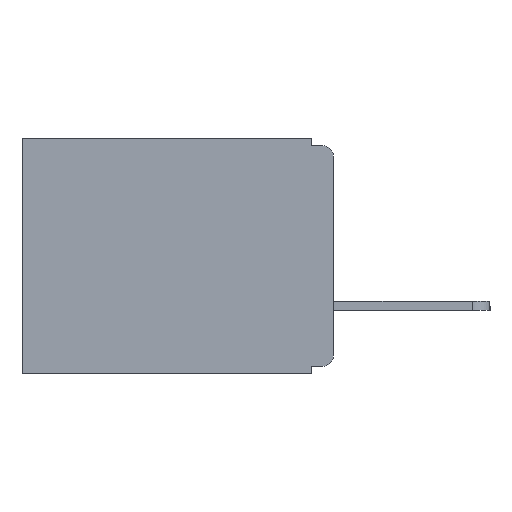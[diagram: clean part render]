
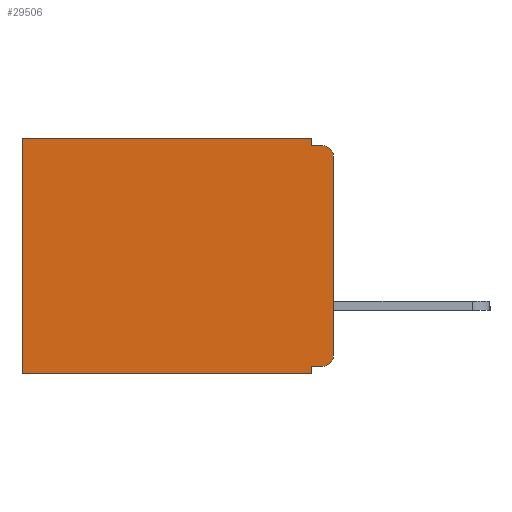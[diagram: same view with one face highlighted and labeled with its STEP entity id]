
A CAD part, left-side view. The second image highlights one B-rep face of the part: STEP entity #29506.
In plain terms, the highlighted planar face has unit normal (-1, 0, 0).
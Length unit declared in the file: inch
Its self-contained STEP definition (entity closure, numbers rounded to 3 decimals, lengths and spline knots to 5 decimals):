
#635 = DIRECTION ( 'NONE',  ( 0., 1., 0. ) ) ;
#1683 = EDGE_CURVE ( 'NONE', #2957, #29857, #15412, .T. ) ;
#1699 = DIRECTION ( 'NONE',  ( 0., 0., -1. ) ) ;
#2133 = CARTESIAN_POINT ( 'NONE',  ( 0.3, 0.015, -0.01 ) ) ;
#2497 = EDGE_CURVE ( 'NONE', #2957, #4548, #22340, .T. ) ;
#2518 = LINE ( 'NONE', #3374, #26071 ) ;
#2524 = VERTEX_POINT ( 'NONE', #17699 ) ;
#2560 = CARTESIAN_POINT ( 'NONE',  ( 0.3, 0.031, -0.32 ) ) ;
#2610 = PLANE ( 'NONE',  #19817 ) ;
#2957 = VERTEX_POINT ( 'NONE', #9171 ) ;
#3186 = ORIENTED_EDGE ( 'NONE', *, *, #26021, .F. ) ;
#3285 = CARTESIAN_POINT ( 'NONE',  ( 0.3, 0.031, -0.33 ) ) ;
#3288 = VERTEX_POINT ( 'NONE', #6997 ) ;
#3374 = CARTESIAN_POINT ( 'NONE',  ( 0.3, 0., -0.33 ) ) ;
#4548 = VERTEX_POINT ( 'NONE', #2560 ) ;
#4597 = VECTOR ( 'NONE', #16615, 39.37008 ) ;
#5363 = CARTESIAN_POINT ( 'NONE',  ( 0.3, 0., 0. ) ) ;
#5438 = VECTOR ( 'NONE', #29386, 39.37008 ) ;
#6080 = LINE ( 'NONE', #25916, #4597 ) ;
#6155 = AXIS2_PLACEMENT_3D ( 'NONE', #29824, #15844, #1699 ) ;
#6926 = ORIENTED_EDGE ( 'NONE', *, *, #22438, .T. ) ;
#6997 = CARTESIAN_POINT ( 'NONE',  ( 0.3, 0.437, -0.33 ) ) ;
#7681 = LINE ( 'NONE', #3285, #12485 ) ;
#8193 = VERTEX_POINT ( 'NONE', #25195 ) ;
#9122 = ORIENTED_EDGE ( 'NONE', *, *, #1683, .T. ) ;
#9171 = CARTESIAN_POINT ( 'NONE',  ( 0.3, 0.015, -0.32 ) ) ;
#9757 = DIRECTION ( 'NONE',  ( 0., 0., -1. ) ) ;
#9834 = VECTOR ( 'NONE', #13675, 39.37008 ) ;
#9893 = LINE ( 'NONE', #5363, #27133 ) ;
#10620 = CARTESIAN_POINT ( 'NONE',  ( 0.3, 0.031, -0.01 ) ) ;
#10645 = ORIENTED_EDGE ( 'NONE', *, *, #26791, .T. ) ;
#11006 = ORIENTED_EDGE ( 'NONE', *, *, #28135, .F. ) ;
#11070 = CARTESIAN_POINT ( 'NONE',  ( 0.3, 0., -0.305 ) ) ;
#11861 = DIRECTION ( 'NONE',  ( 0., 0., -1. ) ) ;
#12472 = EDGE_CURVE ( 'NONE', #14126, #17581, #28627, .T. ) ;
#12485 = VECTOR ( 'NONE', #22163, 39.37008 ) ;
#12557 = VERTEX_POINT ( 'NONE', #18528 ) ;
#12854 = DIRECTION ( 'NONE',  ( -1., 0., 0. ) ) ;
#13504 = EDGE_CURVE ( 'NONE', #30221, #29857, #24241, .T. ) ;
#13516 = CARTESIAN_POINT ( 'NONE',  ( 0.3, 0., -0.01 ) ) ;
#13675 = DIRECTION ( 'NONE',  ( 0., 1., 0. ) ) ;
#13876 = DIRECTION ( 'NONE',  ( 0., 0., -1. ) ) ;
#14126 = VERTEX_POINT ( 'NONE', #10620 ) ;
#14377 = CARTESIAN_POINT ( 'NONE',  ( 0.3, 0., -0.33 ) ) ;
#14617 = LINE ( 'NONE', #23561, #20136 ) ;
#15412 = CIRCLE ( 'NONE', #30006, 0.015 ) ;
#15844 = DIRECTION ( 'NONE',  ( -1., 0., 0. ) ) ;
#16615 = DIRECTION ( 'NONE',  ( 0., 0., -1. ) ) ;
#16975 = VECTOR ( 'NONE', #29858, 39.37008 ) ;
#17057 = CARTESIAN_POINT ( 'NONE',  ( 0.3, 0., -0.32 ) ) ;
#17581 = VERTEX_POINT ( 'NONE', #2133 ) ;
#17671 = CARTESIAN_POINT ( 'NONE',  ( 0.3, 0., -0.33 ) ) ;
#17699 = CARTESIAN_POINT ( 'NONE',  ( 0.3, 0.437, 0. ) ) ;
#18528 = CARTESIAN_POINT ( 'NONE',  ( 0.3, 0.031, 0. ) ) ;
#18924 = EDGE_CURVE ( 'NONE', #2524, #3288, #6080, .T. ) ;
#19273 = FACE_OUTER_BOUND ( 'NONE', #19367, .T. ) ;
#19367 = EDGE_LOOP ( 'NONE', ( #20970, #10645, #22784, #11006, #6926, #23131, #3186, #28190, #21262, #9122 ) ) ;
#19817 = AXIS2_PLACEMENT_3D ( 'NONE', #14377, #23833, #9757 ) ;
#20136 = VECTOR ( 'NONE', #11861, 39.37008 ) ;
#20970 = ORIENTED_EDGE ( 'NONE', *, *, #13504, .F. ) ;
#21262 = ORIENTED_EDGE ( 'NONE', *, *, #2497, .F. ) ;
#22163 = DIRECTION ( 'NONE',  ( 0., 0., -1. ) ) ;
#22340 = LINE ( 'NONE', #17057, #9834 ) ;
#22438 = EDGE_CURVE ( 'NONE', #12557, #2524, #9893, .T. ) ;
#22530 = EDGE_CURVE ( 'NONE', #4548, #8193, #7681, .T. ) ;
#22784 = ORIENTED_EDGE ( 'NONE', *, *, #12472, .F. ) ;
#23131 = ORIENTED_EDGE ( 'NONE', *, *, #18924, .T. ) ;
#23561 = CARTESIAN_POINT ( 'NONE',  ( 0.3, 0.031, 0. ) ) ;
#23833 = DIRECTION ( 'NONE',  ( 1., 0., 0. ) ) ;
#24241 = LINE ( 'NONE', #17671, #5438 ) ;
#24593 = DIRECTION ( 'NONE',  ( 0., 1., 0. ) ) ;
#25195 = CARTESIAN_POINT ( 'NONE',  ( 0.3, 0.031, -0.33 ) ) ;
#25916 = CARTESIAN_POINT ( 'NONE',  ( 0.3, 0.437, -0.33 ) ) ;
#26021 = EDGE_CURVE ( 'NONE', #8193, #3288, #2518, .T. ) ;
#26071 = VECTOR ( 'NONE', #24593, 39.37008 ) ;
#26791 = EDGE_CURVE ( 'NONE', #30221, #17581, #29648, .T. ) ;
#27133 = VECTOR ( 'NONE', #635, 39.37008 ) ;
#27162 = CARTESIAN_POINT ( 'NONE',  ( 0.3, 0.015, -0.305 ) ) ;
#28135 = EDGE_CURVE ( 'NONE', #12557, #14126, #14617, .T. ) ;
#28190 = ORIENTED_EDGE ( 'NONE', *, *, #22530, .F. ) ;
#28627 = LINE ( 'NONE', #13516, #16975 ) ;
#28733 = CARTESIAN_POINT ( 'NONE',  ( 0.3, 0., -0.025 ) ) ;
#29386 = DIRECTION ( 'NONE',  ( 0., 0., -1. ) ) ;
#29506 = ADVANCED_FACE ( 'NONE', ( #19273 ), #2610, .F. ) ;
#29648 = CIRCLE ( 'NONE', #6155, 0.015 ) ;
#29824 = CARTESIAN_POINT ( 'NONE',  ( 0.3, 0.015, -0.025 ) ) ;
#29857 = VERTEX_POINT ( 'NONE', #11070 ) ;
#29858 = DIRECTION ( 'NONE',  ( 0., -1., 0. ) ) ;
#30006 = AXIS2_PLACEMENT_3D ( 'NONE', #27162, #12854, #13876 ) ;
#30221 = VERTEX_POINT ( 'NONE', #28733 ) ;
